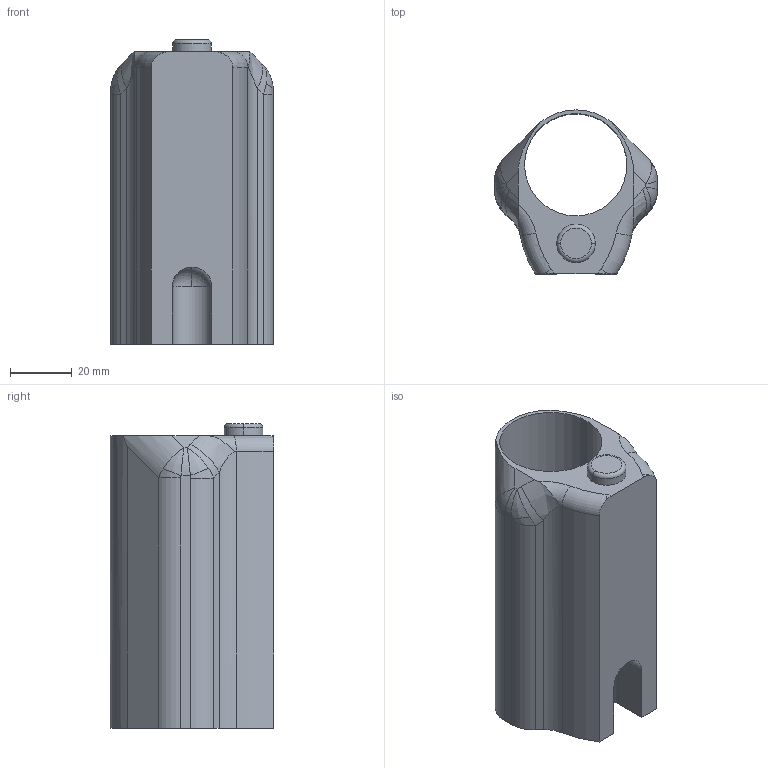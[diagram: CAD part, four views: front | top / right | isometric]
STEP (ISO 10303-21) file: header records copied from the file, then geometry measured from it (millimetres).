
FILE_DESCRIPTION (( 'STEP AP214' ), '1' );
FILE_NAME ('P-15_V2_Part_3.STEP', '2013-12-11T21:50:19', ( 'elpi' ), ( '' ), 'SwSTEP 2.0', 'SolidWorks 2013', '' );
FILE_SCHEMA (( 'AUTOMOTIVE_DESIGN' ));
Length unit declared in the file: inch
Products named in the file (1): P-15_V2_Part_3
Bounding box: 52.54 x 52.84 x 98.28 mm (x, y, z)
Volume: 107315.4 mm3; surface area: 28371 mm2
Topology: 1 solids, 1 shells, 55 faces, 142 edges, 84 vertices
Faces by surface type: cylinder 21, plane 14, bspline 10, torus 8, sphere 2
Entity records: 2159 total; most frequent: CARTESIAN_POINT 856, ORIENTED_EDGE 272, DIRECTION 249, EDGE_CURVE 136, AXIS2_PLACEMENT_3D 99, VERTEX_POINT 84, EDGE_LOOP 58, ADVANCED_FACE 55
